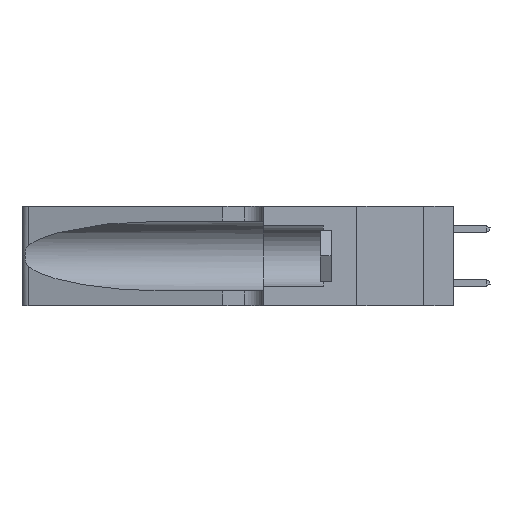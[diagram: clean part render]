
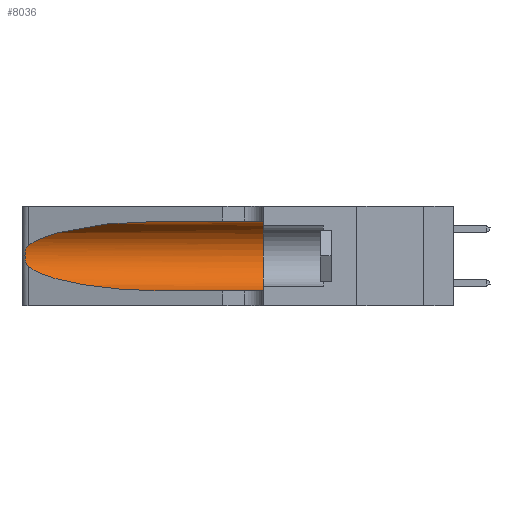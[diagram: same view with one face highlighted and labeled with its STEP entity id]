
A CAD part, left-side view. The second image highlights one B-rep face of the part: STEP entity #8036.
In plain terms, the highlighted cylindrical face has radius 3.308 mm (diameter 6.617 mm), a partial arc.
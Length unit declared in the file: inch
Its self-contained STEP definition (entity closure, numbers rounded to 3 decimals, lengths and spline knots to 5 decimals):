
#139 = CARTESIAN_POINT ( 'NONE',  ( 0.26075, 1.23896, 0.19203 ) ) ;
#1284 = DIRECTION ( 'NONE',  ( 0., -1., 0. ) ) ;
#1408 = EDGE_LOOP ( 'NONE', ( #8612, #14902, #41363, #18010, #3428, #17512 ) ) ;
#2516 = VERTEX_POINT ( 'NONE', #25882 ) ;
#3379 = VERTEX_POINT ( 'NONE', #30022 ) ;
#3428 = ORIENTED_EDGE ( 'NONE', *, *, #3553, .F. ) ;
#3527 = CARTESIAN_POINT ( 'NONE',  ( 0.26017, 1.23833, 0.17102 ) ) ;
#3553 = EDGE_CURVE ( 'NONE', #16849, #35789, #36404, .T. ) ;
#4376 = DIRECTION ( 'NONE',  ( 0., 1., 0. ) ) ;
#5071 = VERTEX_POINT ( 'NONE', #8969 ) ;
#5748 = CARTESIAN_POINT ( 'NONE',  ( 0.25487, 1.22718, 0.22369 ) ) ;
#6883 = CARTESIAN_POINT ( 'NONE',  ( 0.25789, 1.23486, 0.15765 ) ) ;
#8036 = ADVANCED_FACE ( 'NONE', ( #24739 ), #13801, .F. ) ;
#8612 = ORIENTED_EDGE ( 'NONE', *, *, #14749, .T. ) ;
#8969 = CARTESIAN_POINT ( 'NONE',  ( 0.1305, 0.72297, 0.05475 ) ) ;
#10112 = DIRECTION ( 'NONE',  ( 0., -1., 0. ) ) ;
#10120 = CARTESIAN_POINT ( 'NONE',  ( 0.25487, 1.22718, 0.22369 ) ) ;
#10254 = CARTESIAN_POINT ( 'NONE',  ( 0.25555, 1.22993, 0.14849 ) ) ;
#10610 =( BOUNDED_CURVE ( )  B_SPLINE_CURVE ( 3, ( #15660, #38848, #25717, #5748 ),
 .UNSPECIFIED., .F., .F. ) 
 B_SPLINE_CURVE_WITH_KNOTS ( ( 4, 4 ),
 ( 1.5708, 2.84003 ),
 .UNSPECIFIED. ) 
 CURVE ( )  GEOMETRIC_REPRESENTATION_ITEM ( )  RATIONAL_B_SPLINE_CURVE ( ( 1., 0.87, 0.87, 1. ) ) 
 REPRESENTATION_ITEM ( '' )  );
#10949 = EDGE_CURVE ( 'NONE', #2516, #5071, #11352, .T. ) ;
#11352 =( BOUNDED_CURVE ( )  B_SPLINE_CURVE ( 3, ( #29797, #33147, #13217, #36417 ),
 .UNSPECIFIED., .F., .T. ) 
 B_SPLINE_CURVE_WITH_KNOTS ( ( 4, 4 ),
 ( 3.44316, 4.71239 ),
 .UNSPECIFIED. ) 
 CURVE ( )  GEOMETRIC_REPRESENTATION_ITEM ( )  RATIONAL_B_SPLINE_CURVE ( ( 1., 0.87, 0.87, 1. ) ) 
 REPRESENTATION_ITEM ( '' )  );
#11688 = EDGE_CURVE ( 'NONE', #5071, #35789, #29133, .T. ) ;
#13217 = CARTESIAN_POINT ( 'NONE',  ( 0.18966, 0.96281, 0.05475 ) ) ;
#13310 = CARTESIAN_POINT ( 'NONE',  ( 0.1305, 1.61858, 0.05475 ) ) ;
#13801 = CYLINDRICAL_SURFACE ( 'NONE', #27580, 0.13025 ) ;
#14749 = EDGE_CURVE ( 'NONE', #3379, #34046, #10610, .T. ) ;
#14902 = ORIENTED_EDGE ( 'NONE', *, *, #38797, .T. ) ;
#15660 = CARTESIAN_POINT ( 'NONE',  ( 0.1305, 0.72297, 0.31525 ) ) ;
#16043 = AXIS2_PLACEMENT_3D ( 'NONE', #24336, #4376, #27699 ) ;
#16801 = CARTESIAN_POINT ( 'NONE',  ( 0.25787, 1.23484, 0.2124 ) ) ;
#16849 = VERTEX_POINT ( 'NONE', #35740 ) ;
#17512 = ORIENTED_EDGE ( 'NONE', *, *, #37549, .F. ) ;
#18010 = ORIENTED_EDGE ( 'NONE', *, *, #11688, .T. ) ;
#19013 = LINE ( 'NONE', #41125, #24764 ) ;
#20117 = CARTESIAN_POINT ( 'NONE',  ( 0.26018, 1.23835, 0.19895 ) ) ;
#20241 = VECTOR ( 'NONE', #10112, 39.37008 ) ;
#23482 = CARTESIAN_POINT ( 'NONE',  ( 0.26075, 1.23896, 0.178 ) ) ;
#24336 = CARTESIAN_POINT ( 'NONE',  ( 0.1305, 0.35, 0.185 ) ) ;
#24739 = FACE_OUTER_BOUND ( 'NONE', #1408, .T. ) ;
#24764 = VECTOR ( 'NONE', #1284, 39.37008 ) ;
#25389 = CARTESIAN_POINT ( 'NONE',  ( 0.1305, 1.61858, 0.185 ) ) ;
#25717 = CARTESIAN_POINT ( 'NONE',  ( 0.2373, 1.15595, 0.28018 ) ) ;
#25882 = CARTESIAN_POINT ( 'NONE',  ( 0.25487, 1.22718, 0.14631 ) ) ;
#26859 = CARTESIAN_POINT ( 'NONE',  ( 0.25856, 1.23593, 0.16098 ) ) ;
#27580 = AXIS2_PLACEMENT_3D ( 'NONE', #25389, #42013, #28728 ) ;
#27699 = DIRECTION ( 'NONE',  ( 0., 0., 1. ) ) ;
#28728 = DIRECTION ( 'NONE',  ( 0., 0., -1. ) ) ;
#29133 = LINE ( 'NONE', #13310, #20241 ) ;
#29797 = CARTESIAN_POINT ( 'NONE',  ( 0.25487, 1.22718, 0.14631 ) ) ;
#30022 = CARTESIAN_POINT ( 'NONE',  ( 0.1305, 0.72297, 0.31525 ) ) ;
#30175 = CARTESIAN_POINT ( 'NONE',  ( 0.25487, 1.22718, 0.22369 ) ) ;
#30178 = CARTESIAN_POINT ( 'NONE',  ( 0.25639, 1.23186, 0.15144 ) ) ;
#33147 = CARTESIAN_POINT ( 'NONE',  ( 0.2373, 1.15595, 0.08982 ) ) ;
#33372 = CARTESIAN_POINT ( 'NONE',  ( 0.25555, 1.22994, 0.2215 ) ) ;
#33530 = CARTESIAN_POINT ( 'NONE',  ( 0.25487, 1.22718, 0.14631 ) ) ;
#34046 = VERTEX_POINT ( 'NONE', #30175 ) ;
#35201 = CARTESIAN_POINT ( 'NONE',  ( 0.1305, 0.35, 0.05475 ) ) ;
#35740 = CARTESIAN_POINT ( 'NONE',  ( 0.1305, 0.35, 0.31525 ) ) ;
#35789 = VERTEX_POINT ( 'NONE', #35201 ) ;
#36404 = CIRCLE ( 'NONE', #16043, 0.13025 ) ;
#36417 = CARTESIAN_POINT ( 'NONE',  ( 0.1305, 0.72297, 0.05475 ) ) ;
#36667 = CARTESIAN_POINT ( 'NONE',  ( 0.25639, 1.23184, 0.21858 ) ) ;
#37549 = EDGE_CURVE ( 'NONE', #3379, #16849, #19013, .T. ) ;
#38797 = EDGE_CURVE ( 'NONE', #34046, #2516, #39882, .T. ) ;
#38848 = CARTESIAN_POINT ( 'NONE',  ( 0.18966, 0.96281, 0.31525 ) ) ;
#39882 = B_SPLINE_CURVE_WITH_KNOTS ( 'NONE', 3,
 ( #10120, #33372, #36667, #16801, #39983, #20117, #139, #23482, #3527, #26859, #6883, #30178, #10254, #33530 ),
 .UNSPECIFIED., .F., .F.,
 ( 4, 2, 2, 2, 2, 2, 4 ),
 ( 0., 0.00027, 0.00053, 0.00107, 0.0016, 0.00187, 0.00214 ),
 .UNSPECIFIED. ) ;
#39983 = CARTESIAN_POINT ( 'NONE',  ( 0.25854, 1.2359, 0.20912 ) ) ;
#41125 = CARTESIAN_POINT ( 'NONE',  ( 0.1305, 1.61858, 0.31525 ) ) ;
#41363 = ORIENTED_EDGE ( 'NONE', *, *, #10949, .T. ) ;
#42013 = DIRECTION ( 'NONE',  ( 0., -1., 0. ) ) ;
